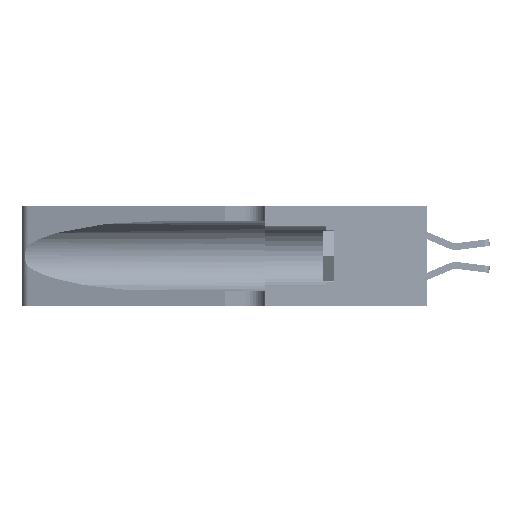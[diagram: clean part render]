
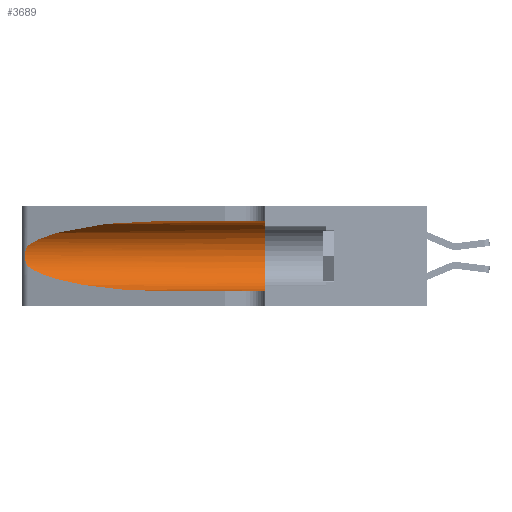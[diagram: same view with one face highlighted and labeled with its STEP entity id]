
A CAD part, left-side view. The second image highlights one B-rep face of the part: STEP entity #3689.
In plain terms, the highlighted cylindrical face has radius 3.308 mm (diameter 6.617 mm), a partial arc.
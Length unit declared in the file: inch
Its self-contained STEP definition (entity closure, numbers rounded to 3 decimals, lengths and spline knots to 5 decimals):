
#112 = VECTOR ( 'NONE', #33766, 39.37008 ) ;
#1202 = LINE ( 'NONE', #30506, #112 ) ;
#1576 = CARTESIAN_POINT ( 'NONE',  ( 0.25639, 1.23184, 0.21858 ) ) ;
#1735 = CARTESIAN_POINT ( 'NONE',  ( 0.2373, 1.15595, 0.28018 ) ) ;
#1979 = FACE_OUTER_BOUND ( 'NONE', #30891, .T. ) ;
#2646 = CARTESIAN_POINT ( 'NONE',  ( 0.25487, 1.22718, 0.22369 ) ) ;
#3200 = DIRECTION ( 'NONE',  ( 0., 0., 1. ) ) ;
#3689 = ADVANCED_FACE ( 'NONE', ( #1979 ), #9975, .F. ) ;
#4052 = VERTEX_POINT ( 'NONE', #11066 ) ;
#5022 = CARTESIAN_POINT ( 'NONE',  ( 0.25854, 1.2359, 0.20912 ) ) ;
#5038 = CARTESIAN_POINT ( 'NONE',  ( 0.18966, 0.96281, 0.31525 ) ) ;
#5597 = DIRECTION ( 'NONE',  ( 0., -1., 0. ) ) ;
#5968 = VECTOR ( 'NONE', #42736, 39.37008 ) ;
#8438 = CARTESIAN_POINT ( 'NONE',  ( 0.26075, 1.23896, 0.19203 ) ) ;
#8978 = CARTESIAN_POINT ( 'NONE',  ( 0.25487, 1.22718, 0.14631 ) ) ;
#9169 = DIRECTION ( 'NONE',  ( 0., 0., -1. ) ) ;
#9975 = CYLINDRICAL_SURFACE ( 'NONE', #37533, 0.13025 ) ;
#10586 = CARTESIAN_POINT ( 'NONE',  ( 0.2373, 1.15595, 0.08982 ) ) ;
#11066 = CARTESIAN_POINT ( 'NONE',  ( 0.1305, 0.35, 0.31525 ) ) ;
#11836 = CARTESIAN_POINT ( 'NONE',  ( 0.26017, 1.23833, 0.17102 ) ) ;
#12852 = CARTESIAN_POINT ( 'NONE',  ( 0.1305, 0.72297, 0.05475 ) ) ;
#14850 = EDGE_CURVE ( 'NONE', #27685, #23261, #1202, .T. ) ;
#14853 = EDGE_CURVE ( 'NONE', #43165, #27685, #40854, .T. ) ;
#15124 = CARTESIAN_POINT ( 'NONE',  ( 0.25555, 1.22994, 0.2215 ) ) ;
#15258 = CARTESIAN_POINT ( 'NONE',  ( 0.25789, 1.23486, 0.15765 ) ) ;
#15857 = CARTESIAN_POINT ( 'NONE',  ( 0.1305, 0.35, 0.05475 ) ) ;
#16262 = EDGE_CURVE ( 'NONE', #23341, #43165, #25516, .T. ) ;
#16762 = CIRCLE ( 'NONE', #37411, 0.13025 ) ;
#17375 = CARTESIAN_POINT ( 'NONE',  ( 0.25487, 1.22718, 0.14631 ) ) ;
#17698 = ORIENTED_EDGE ( 'NONE', *, *, #30877, .T. ) ;
#18625 = CARTESIAN_POINT ( 'NONE',  ( 0.25555, 1.22993, 0.14849 ) ) ;
#21999 = EDGE_CURVE ( 'NONE', #4052, #23261, #16762, .T. ) ;
#22360 =( BOUNDED_CURVE ( )  B_SPLINE_CURVE ( 3, ( #28431, #5038, #1735, #25261 ),
 .UNSPECIFIED., .F., .F. ) 
 B_SPLINE_CURVE_WITH_KNOTS ( ( 4, 4 ),
 ( 1.5708, 2.84003 ),
 .UNSPECIFIED. ) 
 CURVE ( )  GEOMETRIC_REPRESENTATION_ITEM ( )  RATIONAL_B_SPLINE_CURVE ( ( 1., 0.87, 0.87, 1. ) ) 
 REPRESENTATION_ITEM ( '' )  );
#23261 = VERTEX_POINT ( 'NONE', #15857 ) ;
#23341 = VERTEX_POINT ( 'NONE', #2646 ) ;
#23377 = DIRECTION ( 'NONE',  ( 0., 1., 0. ) ) ;
#25107 = CARTESIAN_POINT ( 'NONE',  ( 0.25787, 1.23484, 0.2124 ) ) ;
#25261 = CARTESIAN_POINT ( 'NONE',  ( 0.25487, 1.22718, 0.22369 ) ) ;
#25331 = VERTEX_POINT ( 'NONE', #35569 ) ;
#25455 = ORIENTED_EDGE ( 'NONE', *, *, #21999, .F. ) ;
#25516 = B_SPLINE_CURVE_WITH_KNOTS ( 'NONE', 3,
 ( #38214, #15124, #1576, #25107, #5022, #28419, #8438, #31701, #11836, #34985, #15258, #38354, #18625, #41690 ),
 .UNSPECIFIED., .F., .F.,
 ( 4, 2, 2, 2, 2, 2, 4 ),
 ( 0., 0.00027, 0.00053, 0.00107, 0.0016, 0.00187, 0.00214 ),
 .UNSPECIFIED. ) ;
#26874 = ORIENTED_EDGE ( 'NONE', *, *, #27332, .F. ) ;
#27183 = CARTESIAN_POINT ( 'NONE',  ( 0.18966, 0.96281, 0.05475 ) ) ;
#27332 = EDGE_CURVE ( 'NONE', #25331, #4052, #41359, .T. ) ;
#27685 = VERTEX_POINT ( 'NONE', #12852 ) ;
#28419 = CARTESIAN_POINT ( 'NONE',  ( 0.26018, 1.23835, 0.19895 ) ) ;
#28431 = CARTESIAN_POINT ( 'NONE',  ( 0.1305, 0.72297, 0.31525 ) ) ;
#29119 = CARTESIAN_POINT ( 'NONE',  ( 0.1305, 1.61858, 0.185 ) ) ;
#30506 = CARTESIAN_POINT ( 'NONE',  ( 0.1305, 1.61858, 0.05475 ) ) ;
#30877 = EDGE_CURVE ( 'NONE', #25331, #23341, #22360, .T. ) ;
#30891 = EDGE_LOOP ( 'NONE', ( #17698, #43154, #36741, #43003, #25455, #26874 ) ) ;
#31701 = CARTESIAN_POINT ( 'NONE',  ( 0.26075, 1.23896, 0.178 ) ) ;
#33766 = DIRECTION ( 'NONE',  ( 0., -1., 0. ) ) ;
#34985 = CARTESIAN_POINT ( 'NONE',  ( 0.25856, 1.23593, 0.16098 ) ) ;
#35569 = CARTESIAN_POINT ( 'NONE',  ( 0.1305, 0.72297, 0.31525 ) ) ;
#36741 = ORIENTED_EDGE ( 'NONE', *, *, #14853, .T. ) ;
#37411 = AXIS2_PLACEMENT_3D ( 'NONE', #43133, #23377, #3200 ) ;
#37533 = AXIS2_PLACEMENT_3D ( 'NONE', #29119, #5597, #9169 ) ;
#38214 = CARTESIAN_POINT ( 'NONE',  ( 0.25487, 1.22718, 0.22369 ) ) ;
#38354 = CARTESIAN_POINT ( 'NONE',  ( 0.25639, 1.23186, 0.15144 ) ) ;
#39391 = CARTESIAN_POINT ( 'NONE',  ( 0.1305, 1.61858, 0.31525 ) ) ;
#40452 = CARTESIAN_POINT ( 'NONE',  ( 0.1305, 0.72297, 0.05475 ) ) ;
#40854 =( BOUNDED_CURVE ( )  B_SPLINE_CURVE ( 3, ( #17375, #10586, #27183, #40452 ),
 .UNSPECIFIED., .F., .F. ) 
 B_SPLINE_CURVE_WITH_KNOTS ( ( 4, 4 ),
 ( 3.44316, 4.71239 ),
 .UNSPECIFIED. ) 
 CURVE ( )  GEOMETRIC_REPRESENTATION_ITEM ( )  RATIONAL_B_SPLINE_CURVE ( ( 1., 0.87, 0.87, 1. ) ) 
 REPRESENTATION_ITEM ( '' )  );
#41359 = LINE ( 'NONE', #39391, #5968 ) ;
#41690 = CARTESIAN_POINT ( 'NONE',  ( 0.25487, 1.22718, 0.14631 ) ) ;
#42736 = DIRECTION ( 'NONE',  ( 0., -1., 0. ) ) ;
#43003 = ORIENTED_EDGE ( 'NONE', *, *, #14850, .T. ) ;
#43133 = CARTESIAN_POINT ( 'NONE',  ( 0.1305, 0.35, 0.185 ) ) ;
#43154 = ORIENTED_EDGE ( 'NONE', *, *, #16262, .T. ) ;
#43165 = VERTEX_POINT ( 'NONE', #8978 ) ;
